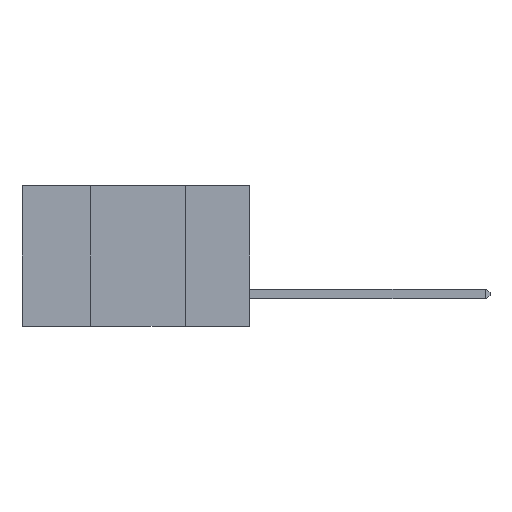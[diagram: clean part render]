
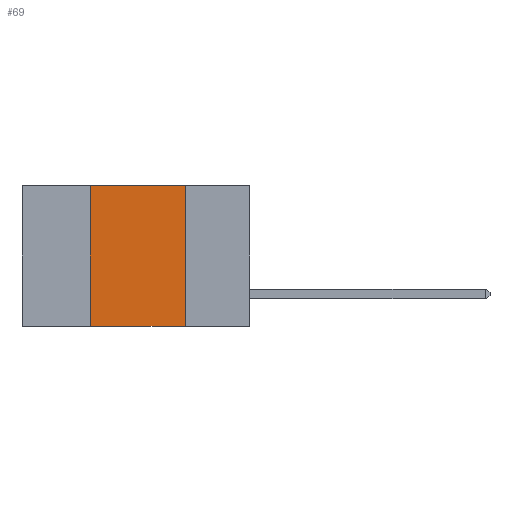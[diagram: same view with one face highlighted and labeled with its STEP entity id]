
A CAD part, left-side view. The second image highlights one B-rep face of the part: STEP entity #69.
In plain terms, the highlighted planar face has unit normal (-1, 0, 0).
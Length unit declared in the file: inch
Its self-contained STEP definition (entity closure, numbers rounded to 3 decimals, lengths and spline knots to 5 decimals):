
#69 = ADVANCED_FACE ( 'NONE', ( #4486 ), #2771, .F. ) ;
#212 = ORIENTED_EDGE ( 'NONE', *, *, #6394, .T. ) ;
#222 = DIRECTION ( 'NONE',  ( 0., 0., 1. ) ) ;
#269 = CARTESIAN_POINT ( 'NONE',  ( 0., 0.42, 0. ) ) ;
#312 = DIRECTION ( 'NONE',  ( 0., -1., 0. ) ) ;
#317 = VECTOR ( 'NONE', #3798, 39.37008 ) ;
#852 = VECTOR ( 'NONE', #312, 39.37008 ) ;
#1799 = DIRECTION ( 'NONE',  ( 0., 0., -1. ) ) ;
#2771 = PLANE ( 'NONE',  #7598 ) ;
#2799 = CARTESIAN_POINT ( 'NONE',  ( 0., 0.42, -0.37 ) ) ;
#3072 = CARTESIAN_POINT ( 'NONE',  ( 0., 0.6, -0.37 ) ) ;
#3465 = LINE ( 'NONE', #3072, #852 ) ;
#3798 = DIRECTION ( 'NONE',  ( 0., 0., -1. ) ) ;
#4486 = FACE_OUTER_BOUND ( 'NONE', #6493, .T. ) ;
#5512 = VERTEX_POINT ( 'NONE', #2799 ) ;
#5775 = VERTEX_POINT ( 'NONE', #269 ) ;
#5838 = CARTESIAN_POINT ( 'NONE',  ( 0., 0.17, -0.37 ) ) ;
#6394 = EDGE_CURVE ( 'NONE', #5512, #10201, #3465, .T. ) ;
#6397 = DIRECTION ( 'NONE',  ( 1., 0., 0. ) ) ;
#6493 = EDGE_LOOP ( 'NONE', ( #12152, #11735, #12301, #212 ) ) ;
#6530 = CARTESIAN_POINT ( 'NONE',  ( 0., 0.6, 0. ) ) ;
#6635 = EDGE_CURVE ( 'NONE', #5775, #8904, #9371, .T. ) ;
#6824 = DIRECTION ( 'NONE',  ( 0., -1., 0. ) ) ;
#7100 = CARTESIAN_POINT ( 'NONE',  ( 0., 0.42, 0. ) ) ;
#7598 = AXIS2_PLACEMENT_3D ( 'NONE', #6530, #6397, #1799 ) ;
#7622 = VECTOR ( 'NONE', #222, 39.37008 ) ;
#8154 = LINE ( 'NONE', #10445, #317 ) ;
#8757 = CARTESIAN_POINT ( 'NONE',  ( 0., 0.6, 0. ) ) ;
#8904 = VERTEX_POINT ( 'NONE', #11942 ) ;
#9062 = EDGE_CURVE ( 'NONE', #8904, #10201, #8154, .T. ) ;
#9069 = VECTOR ( 'NONE', #6824, 39.37008 ) ;
#9371 = LINE ( 'NONE', #8757, #9069 ) ;
#9756 = EDGE_CURVE ( 'NONE', #5512, #5775, #10910, .T. ) ;
#10201 = VERTEX_POINT ( 'NONE', #5838 ) ;
#10445 = CARTESIAN_POINT ( 'NONE',  ( 0., 0.17, 0. ) ) ;
#10910 = LINE ( 'NONE', #7100, #7622 ) ;
#11735 = ORIENTED_EDGE ( 'NONE', *, *, #6635, .F. ) ;
#11942 = CARTESIAN_POINT ( 'NONE',  ( 0., 0.17, 0. ) ) ;
#12152 = ORIENTED_EDGE ( 'NONE', *, *, #9062, .F. ) ;
#12301 = ORIENTED_EDGE ( 'NONE', *, *, #9756, .F. ) ;
